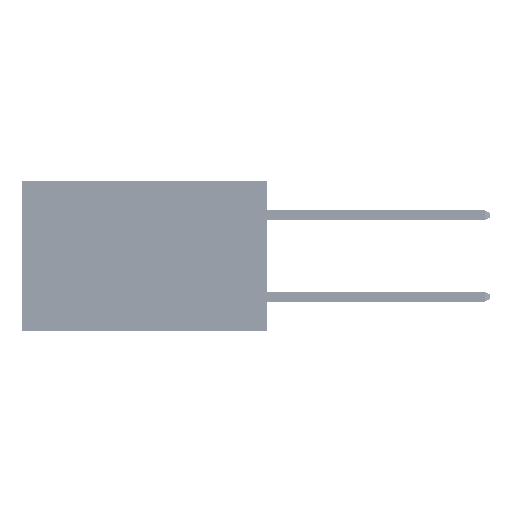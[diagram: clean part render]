
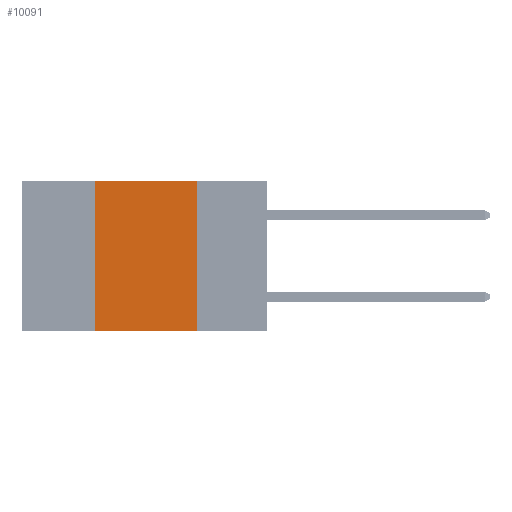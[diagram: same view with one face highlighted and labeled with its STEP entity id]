
A CAD part, left-side view. The second image highlights one B-rep face of the part: STEP entity #10091.
In plain terms, the highlighted planar face has unit normal (-1, 0, 0).
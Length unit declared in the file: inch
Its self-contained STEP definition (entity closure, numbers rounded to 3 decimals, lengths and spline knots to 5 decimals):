
#1746 = LINE ( 'NONE', #19646, #21610 ) ;
#2446 = FACE_OUTER_BOUND ( 'NONE', #41034, .T. ) ;
#4809 = VECTOR ( 'NONE', #41097, 39.37008 ) ;
#5624 = CARTESIAN_POINT ( 'NONE',  ( 0., 0.6, 0. ) ) ;
#6133 = LINE ( 'NONE', #7640, #11177 ) ;
#6614 = VECTOR ( 'NONE', #16535, 39.37008 ) ;
#7640 = CARTESIAN_POINT ( 'NONE',  ( 0., 0.6, 0. ) ) ;
#8223 = VERTEX_POINT ( 'NONE', #44828 ) ;
#8950 = DIRECTION ( 'NONE',  ( 0., 0., -1. ) ) ;
#9837 = CARTESIAN_POINT ( 'NONE',  ( 0., 0.6, -0.37 ) ) ;
#9922 = CARTESIAN_POINT ( 'NONE',  ( 0., 0.42, 0. ) ) ;
#10091 = ADVANCED_FACE ( 'NONE', ( #2446 ), #17467, .F. ) ;
#11177 = VECTOR ( 'NONE', #27197, 39.37008 ) ;
#12046 = ORIENTED_EDGE ( 'NONE', *, *, #15408, .F. ) ;
#14477 = VERTEX_POINT ( 'NONE', #41053 ) ;
#15408 = EDGE_CURVE ( 'NONE', #49729, #40092, #1746, .T. ) ;
#16125 = EDGE_CURVE ( 'NONE', #14477, #8223, #38807, .T. ) ;
#16398 = ORIENTED_EDGE ( 'NONE', *, *, #23329, .F. ) ;
#16535 = DIRECTION ( 'NONE',  ( 0., 0., -1. ) ) ;
#17467 = PLANE ( 'NONE',  #44105 ) ;
#18105 = ORIENTED_EDGE ( 'NONE', *, *, #16125, .F. ) ;
#19646 = CARTESIAN_POINT ( 'NONE',  ( 0., 0.42, 0. ) ) ;
#21610 = VECTOR ( 'NONE', #51189, 39.37008 ) ;
#23329 = EDGE_CURVE ( 'NONE', #40092, #14477, #6133, .T. ) ;
#27135 = LINE ( 'NONE', #9837, #4809 ) ;
#27197 = DIRECTION ( 'NONE',  ( 0., -1., 0. ) ) ;
#32573 = CARTESIAN_POINT ( 'NONE',  ( 0., 0.17, 0. ) ) ;
#33792 = CARTESIAN_POINT ( 'NONE',  ( 0., 0.42, -0.37 ) ) ;
#35116 = EDGE_CURVE ( 'NONE', #49729, #8223, #27135, .T. ) ;
#38807 = LINE ( 'NONE', #32573, #6614 ) ;
#40092 = VERTEX_POINT ( 'NONE', #9922 ) ;
#40393 = DIRECTION ( 'NONE',  ( 1., 0., 0. ) ) ;
#41034 = EDGE_LOOP ( 'NONE', ( #18105, #16398, #12046, #46421 ) ) ;
#41053 = CARTESIAN_POINT ( 'NONE',  ( 0., 0.17, 0. ) ) ;
#41097 = DIRECTION ( 'NONE',  ( 0., -1., 0. ) ) ;
#44105 = AXIS2_PLACEMENT_3D ( 'NONE', #5624, #40393, #8950 ) ;
#44828 = CARTESIAN_POINT ( 'NONE',  ( 0., 0.17, -0.37 ) ) ;
#46421 = ORIENTED_EDGE ( 'NONE', *, *, #35116, .T. ) ;
#49729 = VERTEX_POINT ( 'NONE', #33792 ) ;
#51189 = DIRECTION ( 'NONE',  ( 0., 0., 1. ) ) ;
